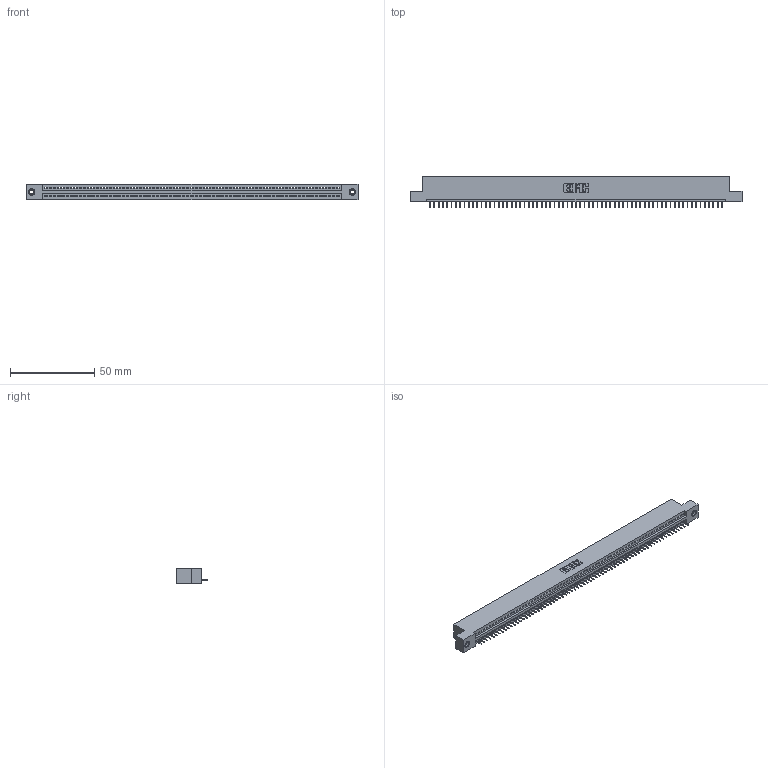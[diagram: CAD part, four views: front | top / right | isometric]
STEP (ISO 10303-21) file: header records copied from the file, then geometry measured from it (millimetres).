
FILE_DESCRIPTION (( 'STEP AP203' ), '1' );
FILE_NAME ('395-069-525-108.STEP', '2020-09-25T04:20:32', ( '' ), ( '' ), 'SwSTEP 2.0', 'SolidWorks 2020', '' );
FILE_SCHEMA (( 'CONFIG_CONTROL_DESIGN' ));
Length unit declared in the file: inch
Products named in the file (4): 345-250-001_345-250-003-102; 345 Part_Flush Mounting Lugs - 0.156 Dia-TI; 395-069-525-108; 345-292-001_345-293-125
Assembly tree (72 placements, depth 2):
  395-069-525-108
    345 Part_Flush Mounting Lugs - 0.156 Dia-TI
    345-292-001_345-293-125  x69
    345-250-001_345-250-003-102  x2
Bounding box: 196.47 x 18.72 x 9.4 mm (x, y, z)
Volume: 18593.8 mm3; surface area: 24156.1 mm2
Topology: 72 solids, 72 shells, 4464 faces, 12897 edges, 8314 vertices
Faces by surface type: plane 3286, cylinder 1162, cone 12, torus 4
Entity records: 49556 total; most frequent: CARTESIAN_POINT 8562, ORIENTED_EDGE 8558, DIRECTION 7467, EDGE_CURVE 4279, LINE 3855, VECTOR 3855, VERTEX_POINT 2844, AXIS2_PLACEMENT_3D 1806
